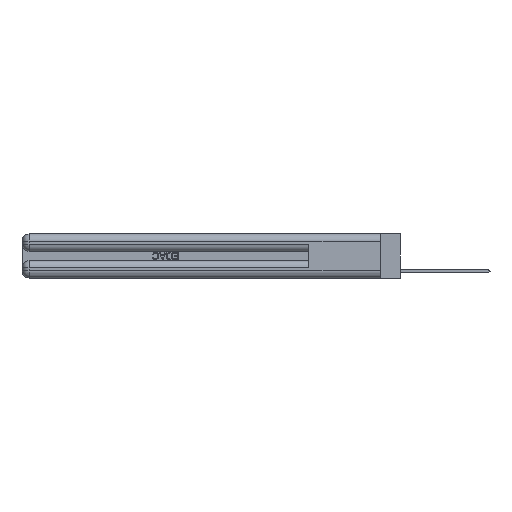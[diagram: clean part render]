
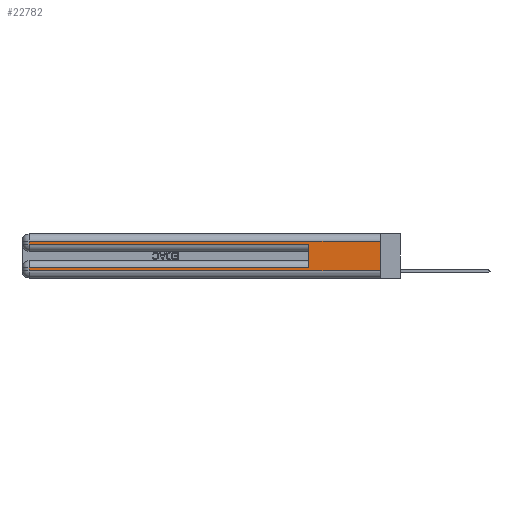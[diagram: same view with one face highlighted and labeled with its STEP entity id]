
A CAD part, left-side view. The second image highlights one B-rep face of the part: STEP entity #22782.
In plain terms, the highlighted planar face has unit normal (-1, 0, 0).
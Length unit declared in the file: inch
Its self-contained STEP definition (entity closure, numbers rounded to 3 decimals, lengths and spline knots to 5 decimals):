
#84 = CARTESIAN_POINT ( 'NONE',  ( 0., 2.94, 0.085 ) ) ;
#107 = EDGE_CURVE ( 'NONE', #18984, #24873, #21978, .T. ) ;
#551 = EDGE_CURVE ( 'NONE', #9178, #18984, #2999, .T. ) ;
#983 = DIRECTION ( 'NONE',  ( 1., 0., 0. ) ) ;
#1239 = ORIENTED_EDGE ( 'NONE', *, *, #107, .T. ) ;
#2999 = LINE ( 'NONE', #29334, #9012 ) ;
#3403 = CARTESIAN_POINT ( 'NONE',  ( 0., 2.94, 0.06 ) ) ;
#3574 = CARTESIAN_POINT ( 'NONE',  ( 0., 0.6, 0.145 ) ) ;
#4071 = EDGE_LOOP ( 'NONE', ( #30702, #20589, #6293, #1239, #11482, #15178, #12444, #15605 ) ) ;
#4151 = CARTESIAN_POINT ( 'NONE',  ( 0., 2.94, 0.31 ) ) ;
#4661 = VECTOR ( 'NONE', #26746, 39.37008 ) ;
#5330 = CARTESIAN_POINT ( 'NONE',  ( 0., 0., 0.085 ) ) ;
#5418 = CARTESIAN_POINT ( 'NONE',  ( 0., 2.94, 0.37 ) ) ;
#5827 = CARTESIAN_POINT ( 'NONE',  ( 0., 0., 0.37 ) ) ;
#5917 = EDGE_CURVE ( 'NONE', #14922, #9871, #10426, .T. ) ;
#6293 = ORIENTED_EDGE ( 'NONE', *, *, #551, .T. ) ;
#6560 = DIRECTION ( 'NONE',  ( 0., 0., -1. ) ) ;
#6749 = VERTEX_POINT ( 'NONE', #3403 ) ;
#7159 = VERTEX_POINT ( 'NONE', #84 ) ;
#7595 = VECTOR ( 'NONE', #15535, 39.37008 ) ;
#9012 = VECTOR ( 'NONE', #6560, 39.37008 ) ;
#9178 = VERTEX_POINT ( 'NONE', #4151 ) ;
#9824 = CARTESIAN_POINT ( 'NONE',  ( 0., 0.6, 0.285 ) ) ;
#9871 = VERTEX_POINT ( 'NONE', #20449 ) ;
#10426 = LINE ( 'NONE', #5827, #30185 ) ;
#11468 = LINE ( 'NONE', #3574, #4661 ) ;
#11482 = ORIENTED_EDGE ( 'NONE', *, *, #27531, .F. ) ;
#12365 = LINE ( 'NONE', #5418, #19657 ) ;
#12444 = ORIENTED_EDGE ( 'NONE', *, *, #29748, .T. ) ;
#12782 = DIRECTION ( 'NONE',  ( 0., -1., 0. ) ) ;
#13100 = CARTESIAN_POINT ( 'NONE',  ( 0., 0., 0.285 ) ) ;
#13274 = DIRECTION ( 'NONE',  ( 0., 1., 0. ) ) ;
#13446 = VERTEX_POINT ( 'NONE', #26823 ) ;
#14338 = EDGE_CURVE ( 'NONE', #14922, #9178, #28967, .T. ) ;
#14922 = VERTEX_POINT ( 'NONE', #23427 ) ;
#15178 = ORIENTED_EDGE ( 'NONE', *, *, #25073, .T. ) ;
#15535 = DIRECTION ( 'NONE',  ( 0., 1., 0. ) ) ;
#15605 = ORIENTED_EDGE ( 'NONE', *, *, #19838, .T. ) ;
#16364 = CARTESIAN_POINT ( 'NONE',  ( 0., 0., 0.37 ) ) ;
#16696 = VECTOR ( 'NONE', #12782, 39.37008 ) ;
#18984 = VERTEX_POINT ( 'NONE', #22843 ) ;
#19657 = VECTOR ( 'NONE', #26127, 39.37008 ) ;
#19838 = EDGE_CURVE ( 'NONE', #6749, #9871, #24973, .T. ) ;
#20449 = CARTESIAN_POINT ( 'NONE',  ( 0., 0., 0.06 ) ) ;
#20589 = ORIENTED_EDGE ( 'NONE', *, *, #14338, .T. ) ;
#21556 = CARTESIAN_POINT ( 'NONE',  ( 0., 0., 0.06 ) ) ;
#21911 = FACE_OUTER_BOUND ( 'NONE', #4071, .T. ) ;
#21978 = LINE ( 'NONE', #13100, #16696 ) ;
#22782 = ADVANCED_FACE ( 'NONE', ( #21911 ), #31720, .F. ) ;
#22843 = CARTESIAN_POINT ( 'NONE',  ( 0., 2.94, 0.285 ) ) ;
#23150 = AXIS2_PLACEMENT_3D ( 'NONE', #16364, #983, #26754 ) ;
#23427 = CARTESIAN_POINT ( 'NONE',  ( 0., 0., 0.31 ) ) ;
#24562 = VECTOR ( 'NONE', #13274, 39.37008 ) ;
#24873 = VERTEX_POINT ( 'NONE', #9824 ) ;
#24973 = LINE ( 'NONE', #21556, #29389 ) ;
#25073 = EDGE_CURVE ( 'NONE', #13446, #7159, #32195, .T. ) ;
#26127 = DIRECTION ( 'NONE',  ( 0., 0., -1. ) ) ;
#26709 = DIRECTION ( 'NONE',  ( 0., -1., 0. ) ) ;
#26746 = DIRECTION ( 'NONE',  ( 0., 0., 1. ) ) ;
#26754 = DIRECTION ( 'NONE',  ( 0., 0., -1. ) ) ;
#26763 = DIRECTION ( 'NONE',  ( 0., 0., -1. ) ) ;
#26823 = CARTESIAN_POINT ( 'NONE',  ( 0., 0.6, 0.085 ) ) ;
#27531 = EDGE_CURVE ( 'NONE', #13446, #24873, #11468, .T. ) ;
#28967 = LINE ( 'NONE', #30993, #7595 ) ;
#29334 = CARTESIAN_POINT ( 'NONE',  ( 0., 2.94, 0.37 ) ) ;
#29389 = VECTOR ( 'NONE', #26709, 39.37008 ) ;
#29748 = EDGE_CURVE ( 'NONE', #7159, #6749, #12365, .T. ) ;
#30185 = VECTOR ( 'NONE', #26763, 39.37008 ) ;
#30702 = ORIENTED_EDGE ( 'NONE', *, *, #5917, .F. ) ;
#30993 = CARTESIAN_POINT ( 'NONE',  ( 0., 0., 0.31 ) ) ;
#31720 = PLANE ( 'NONE',  #23150 ) ;
#32195 = LINE ( 'NONE', #5330, #24562 ) ;
